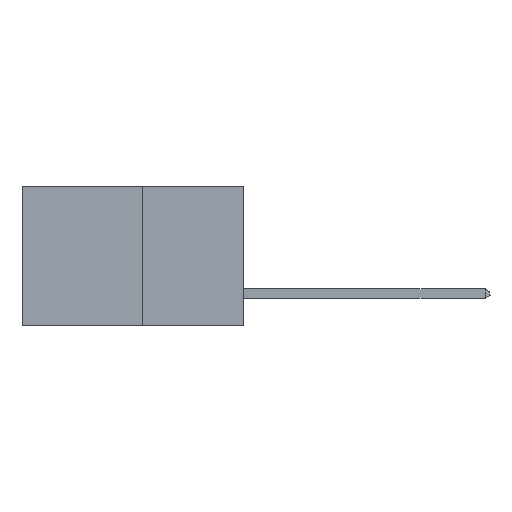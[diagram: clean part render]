
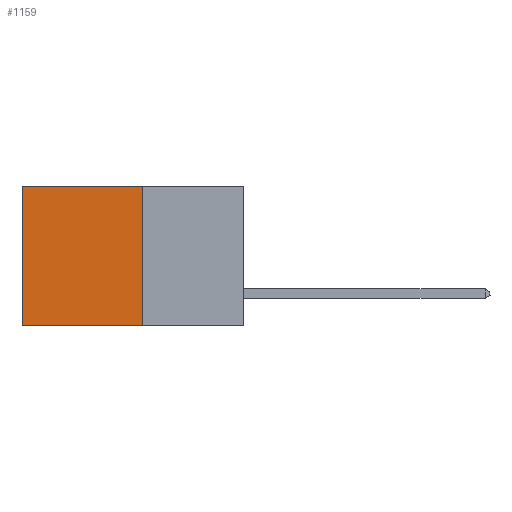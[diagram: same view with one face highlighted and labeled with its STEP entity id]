
A CAD part, left-side view. The second image highlights one B-rep face of the part: STEP entity #1159.
In plain terms, the highlighted planar face has unit normal (-1, 0, 0).
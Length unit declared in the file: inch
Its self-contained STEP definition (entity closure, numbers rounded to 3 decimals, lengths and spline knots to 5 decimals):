
#12 = DIRECTION ( 'NONE',  ( 1., 0., 0. ) ) ;
#360 = VECTOR ( 'NONE', #802, 39.37008 ) ;
#444 = LINE ( 'NONE', #3267, #8145 ) ;
#497 = ORIENTED_EDGE ( 'NONE', *, *, #7060, .T. ) ;
#802 = DIRECTION ( 'NONE',  ( 0., 1., 0. ) ) ;
#1125 = CARTESIAN_POINT ( 'NONE',  ( 0.277, 0.59, -0.37 ) ) ;
#1159 = ADVANCED_FACE ( 'NONE', ( #6860 ), #4688, .F. ) ;
#1652 = CARTESIAN_POINT ( 'NONE',  ( 0.277, 0.27, 0. ) ) ;
#2320 = LINE ( 'NONE', #2837, #6918 ) ;
#2837 = CARTESIAN_POINT ( 'NONE',  ( 0.277, 0.27, -0.37 ) ) ;
#3267 = CARTESIAN_POINT ( 'NONE',  ( 0.277, 0.27, -0.37 ) ) ;
#3389 = LINE ( 'NONE', #1652, #360 ) ;
#3958 = CARTESIAN_POINT ( 'NONE',  ( 0.277, 0.27, -0.37 ) ) ;
#4688 = PLANE ( 'NONE',  #5193 ) ;
#5159 = DIRECTION ( 'NONE',  ( 0., 1., 0. ) ) ;
#5191 = LINE ( 'NONE', #1125, #7413 ) ;
#5193 = AXIS2_PLACEMENT_3D ( 'NONE', #3958, #12, #9975 ) ;
#5716 = ORIENTED_EDGE ( 'NONE', *, *, #8491, .F. ) ;
#5721 = VERTEX_POINT ( 'NONE', #10372 ) ;
#6860 = FACE_OUTER_BOUND ( 'NONE', #7030, .T. ) ;
#6918 = VECTOR ( 'NONE', #11226, 39.37008 ) ;
#7030 = EDGE_LOOP ( 'NONE', ( #7907, #10365, #5716, #497 ) ) ;
#7060 = EDGE_CURVE ( 'NONE', #11167, #9017, #3389, .T. ) ;
#7413 = VECTOR ( 'NONE', #10806, 39.37008 ) ;
#7907 = ORIENTED_EDGE ( 'NONE', *, *, #10201, .T. ) ;
#8145 = VECTOR ( 'NONE', #5159, 39.37008 ) ;
#8491 = EDGE_CURVE ( 'NONE', #11167, #5721, #2320, .T. ) ;
#8808 = EDGE_CURVE ( 'NONE', #5721, #11015, #444, .T. ) ;
#9017 = VERTEX_POINT ( 'NONE', #10480 ) ;
#9355 = CARTESIAN_POINT ( 'NONE',  ( 0.277, 0.27, 0. ) ) ;
#9925 = CARTESIAN_POINT ( 'NONE',  ( 0.277, 0.59, -0.37 ) ) ;
#9975 = DIRECTION ( 'NONE',  ( 0., 0., -1. ) ) ;
#10201 = EDGE_CURVE ( 'NONE', #9017, #11015, #5191, .T. ) ;
#10365 = ORIENTED_EDGE ( 'NONE', *, *, #8808, .F. ) ;
#10372 = CARTESIAN_POINT ( 'NONE',  ( 0.277, 0.27, -0.37 ) ) ;
#10480 = CARTESIAN_POINT ( 'NONE',  ( 0.277, 0.59, 0. ) ) ;
#10806 = DIRECTION ( 'NONE',  ( 0., 0., -1. ) ) ;
#11015 = VERTEX_POINT ( 'NONE', #9925 ) ;
#11167 = VERTEX_POINT ( 'NONE', #9355 ) ;
#11226 = DIRECTION ( 'NONE',  ( 0., 0., -1. ) ) ;
